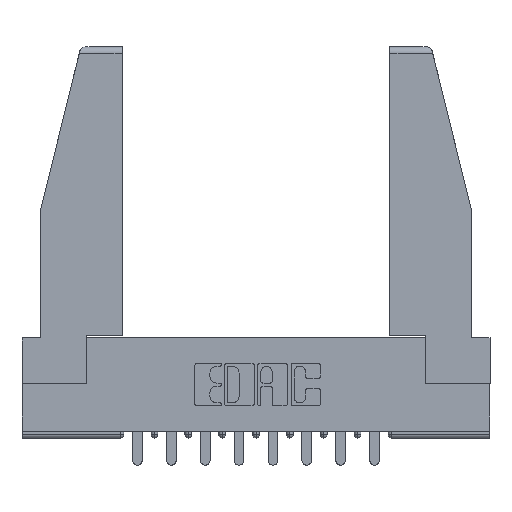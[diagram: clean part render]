
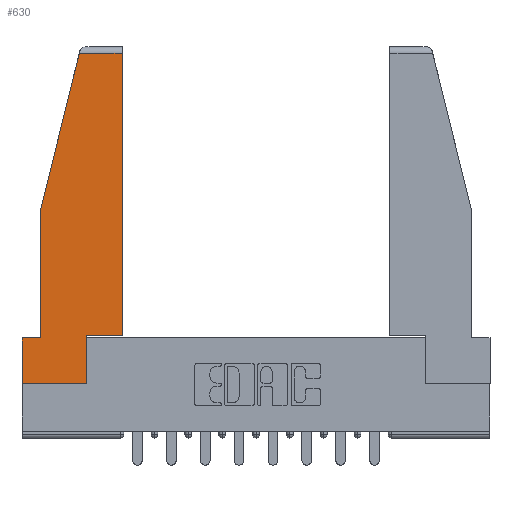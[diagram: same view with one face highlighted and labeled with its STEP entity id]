
A CAD part, top view. The second image highlights one B-rep face of the part: STEP entity #630.
In plain terms, the highlighted planar face has unit normal (0, 0, 1).
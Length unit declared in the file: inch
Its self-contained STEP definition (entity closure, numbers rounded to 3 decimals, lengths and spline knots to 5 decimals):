
#630 = ADVANCED_FACE ( 'NONE', ( #10306 ), #3740, .T. ) ;
#755 = ORIENTED_EDGE ( 'NONE', *, *, #5987, .T. ) ;
#776 = DIRECTION ( 'NONE',  ( 1., 0., 0. ) ) ;
#952 = VECTOR ( 'NONE', #10526, 39.37008 ) ;
#1040 = CARTESIAN_POINT ( 'NONE',  ( 0., 0.21, 0. ) ) ;
#1368 = DIRECTION ( 'NONE',  ( 0., 0., 1. ) ) ;
#1487 = VERTEX_POINT ( 'NONE', #3109 ) ;
#1496 = CARTESIAN_POINT ( 'NONE',  ( 0., 1.52, 0. ) ) ;
#1963 = VECTOR ( 'NONE', #14015, 39.37008 ) ;
#2250 = CARTESIAN_POINT ( 'NONE',  ( 0.086, 0.8, 0. ) ) ;
#2486 = VERTEX_POINT ( 'NONE', #12763 ) ;
#3109 = CARTESIAN_POINT ( 'NONE',  ( 0.461, 1.52, 0. ) ) ;
#3131 = ORIENTED_EDGE ( 'NONE', *, *, #8168, .T. ) ;
#3344 = LINE ( 'NONE', #2250, #11217 ) ;
#3497 = VECTOR ( 'NONE', #5153, 39.37008 ) ;
#3635 = CARTESIAN_POINT ( 'NONE',  ( 0.297, 0.223, 0. ) ) ;
#3740 = PLANE ( 'NONE',  #10579 ) ;
#4025 = EDGE_LOOP ( 'NONE', ( #6957, #12000, #12735, #13519, #755, #11092, #8115, #3131, #11791 ) ) ;
#4460 = VECTOR ( 'NONE', #9962, 39.37008 ) ;
#4531 = CARTESIAN_POINT ( 'NONE',  ( 0.297, 0., 0. ) ) ;
#4785 = VECTOR ( 'NONE', #14924, 39.37008 ) ;
#4983 = EDGE_CURVE ( 'NONE', #9511, #5496, #6357, .T. ) ;
#5153 = DIRECTION ( 'NONE',  ( 0., 1., 0. ) ) ;
#5210 = EDGE_CURVE ( 'NONE', #1487, #14212, #11412, .T. ) ;
#5312 = CARTESIAN_POINT ( 'NONE',  ( 0., 0., 0. ) ) ;
#5346 = CARTESIAN_POINT ( 'NONE',  ( 0., 0.21, 0. ) ) ;
#5362 = LINE ( 'NONE', #6362, #3497 ) ;
#5462 = EDGE_CURVE ( 'NONE', #8687, #11457, #8317, .T. ) ;
#5496 = VERTEX_POINT ( 'NONE', #12907 ) ;
#5647 = LINE ( 'NONE', #4531, #1963 ) ;
#5759 = CARTESIAN_POINT ( 'NONE',  ( 0.271, 1.55, 0. ) ) ;
#5831 = EDGE_CURVE ( 'NONE', #5496, #1487, #5362, .T. ) ;
#5866 = LINE ( 'NONE', #1040, #4785 ) ;
#5987 = EDGE_CURVE ( 'NONE', #10796, #2486, #9191, .T. ) ;
#6357 = LINE ( 'NONE', #13942, #12940 ) ;
#6362 = CARTESIAN_POINT ( 'NONE',  ( 0.461, 0.223, 0. ) ) ;
#6957 = ORIENTED_EDGE ( 'NONE', *, *, #5831, .T. ) ;
#6997 = EDGE_CURVE ( 'NONE', #2486, #8687, #5866, .T. ) ;
#7015 = LINE ( 'NONE', #5759, #952 ) ;
#7692 = CARTESIAN_POINT ( 'NONE',  ( 0.086, 0.8, 0. ) ) ;
#7836 = DIRECTION ( 'NONE',  ( -1., 0., 0. ) ) ;
#8089 = CARTESIAN_POINT ( 'NONE',  ( 0.2636, 1.52, 0. ) ) ;
#8115 = ORIENTED_EDGE ( 'NONE', *, *, #5462, .T. ) ;
#8168 = EDGE_CURVE ( 'NONE', #11457, #9511, #5647, .T. ) ;
#8317 = LINE ( 'NONE', #5312, #8854 ) ;
#8687 = VERTEX_POINT ( 'NONE', #13644 ) ;
#8854 = VECTOR ( 'NONE', #776, 39.37008 ) ;
#9094 = VERTEX_POINT ( 'NONE', #7692 ) ;
#9191 = LINE ( 'NONE', #5346, #11011 ) ;
#9358 = DIRECTION ( 'NONE',  ( 1., 0., 0. ) ) ;
#9511 = VERTEX_POINT ( 'NONE', #3635 ) ;
#9962 = DIRECTION ( 'NONE',  ( -1., 0., 0. ) ) ;
#10156 = CARTESIAN_POINT ( 'NONE',  ( 0.297, 0., 0. ) ) ;
#10306 = FACE_OUTER_BOUND ( 'NONE', #4025, .T. ) ;
#10526 = DIRECTION ( 'NONE',  ( -0.239, -0.971, 0. ) ) ;
#10579 = AXIS2_PLACEMENT_3D ( 'NONE', #11910, #1368, #14220 ) ;
#10796 = VERTEX_POINT ( 'NONE', #13269 ) ;
#11011 = VECTOR ( 'NONE', #7836, 39.37008 ) ;
#11092 = ORIENTED_EDGE ( 'NONE', *, *, #6997, .T. ) ;
#11217 = VECTOR ( 'NONE', #13933, 39.37008 ) ;
#11412 = LINE ( 'NONE', #1496, #4460 ) ;
#11457 = VERTEX_POINT ( 'NONE', #10156 ) ;
#11477 = EDGE_CURVE ( 'NONE', #9094, #10796, #3344, .T. ) ;
#11583 = EDGE_CURVE ( 'NONE', #14212, #9094, #7015, .T. ) ;
#11791 = ORIENTED_EDGE ( 'NONE', *, *, #4983, .T. ) ;
#11910 = CARTESIAN_POINT ( 'NONE',  ( 0., 0., 0. ) ) ;
#12000 = ORIENTED_EDGE ( 'NONE', *, *, #5210, .T. ) ;
#12735 = ORIENTED_EDGE ( 'NONE', *, *, #11583, .T. ) ;
#12763 = CARTESIAN_POINT ( 'NONE',  ( 0., 0.21, 0. ) ) ;
#12907 = CARTESIAN_POINT ( 'NONE',  ( 0.461, 0.223, 0. ) ) ;
#12940 = VECTOR ( 'NONE', #9358, 39.37008 ) ;
#13269 = CARTESIAN_POINT ( 'NONE',  ( 0.086, 0.21, 0. ) ) ;
#13519 = ORIENTED_EDGE ( 'NONE', *, *, #11477, .T. ) ;
#13644 = CARTESIAN_POINT ( 'NONE',  ( 0., 0., 0. ) ) ;
#13933 = DIRECTION ( 'NONE',  ( 0., -1., 0. ) ) ;
#13942 = CARTESIAN_POINT ( 'NONE',  ( 0.297, 0.223, 0. ) ) ;
#14015 = DIRECTION ( 'NONE',  ( 0., 1., 0. ) ) ;
#14212 = VERTEX_POINT ( 'NONE', #8089 ) ;
#14220 = DIRECTION ( 'NONE',  ( 1., 0., 0. ) ) ;
#14924 = DIRECTION ( 'NONE',  ( 0., -1., 0. ) ) ;
